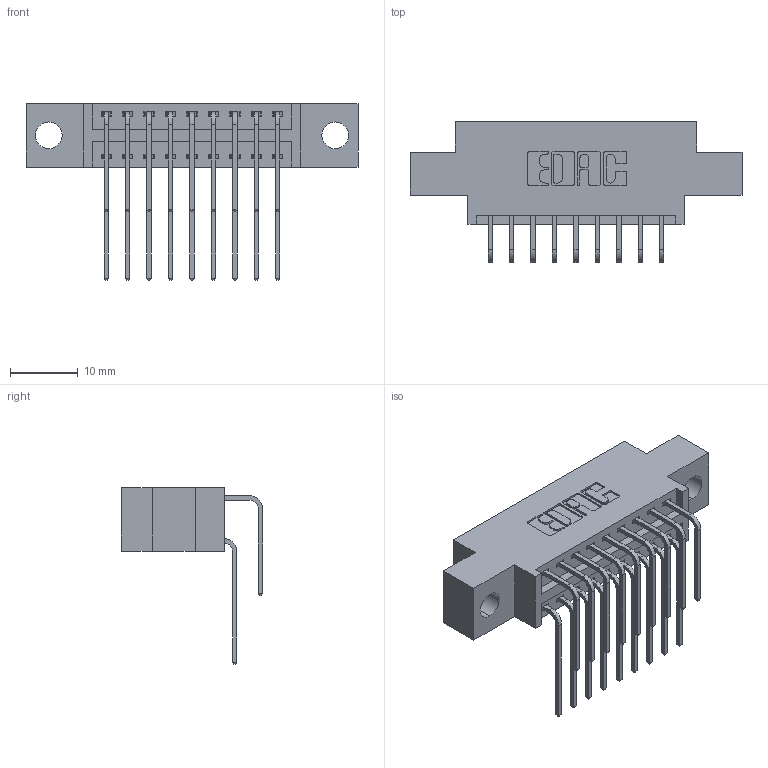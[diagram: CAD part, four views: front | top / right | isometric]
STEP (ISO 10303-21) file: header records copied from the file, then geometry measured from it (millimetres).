
FILE_DESCRIPTION (( 'STEP AP203' ), '1' );
FILE_NAME ('346-018-559-804.STEP', '2022-05-18T18:16:11', ( '' ), ( '' ), 'SwSTEP 2.0', 'SolidWorks 2020', '' );
FILE_SCHEMA (( 'CONFIG_CONTROL_DESIGN' ));
Length unit declared in the file: inch
Products named in the file (4): 346 Part_0.170 Offset - 0.156 Dia-TH; 345-292-001_558 559 Tail - 1; 345-292-001_559 Tail - 2; 346-018-559-804
Assembly tree (19 placements, depth 2):
  346-018-559-804
    346 Part_0.170 Offset - 0.156 Dia-TH
    345-292-001_558 559 Tail - 1  x9
    345-292-001_559 Tail - 2  x9
Bounding box: 49.15 x 20.89 x 26.16 mm (x, y, z)
Volume: 4379.6 mm3; surface area: 6027 mm2
Topology: 19 solids, 19 shells, 1112 faces, 3275 edges, 2158 vertices
Faces by surface type: plane 760, cylinder 352
Entity records: 12651 total; most frequent: CARTESIAN_POINT 2189, ORIENTED_EDGE 2070, DIRECTION 1951, EDGE_CURVE 1035, LINE 827, VECTOR 827, VERTEX_POINT 686, AXIS2_PLACEMENT_3D 562
